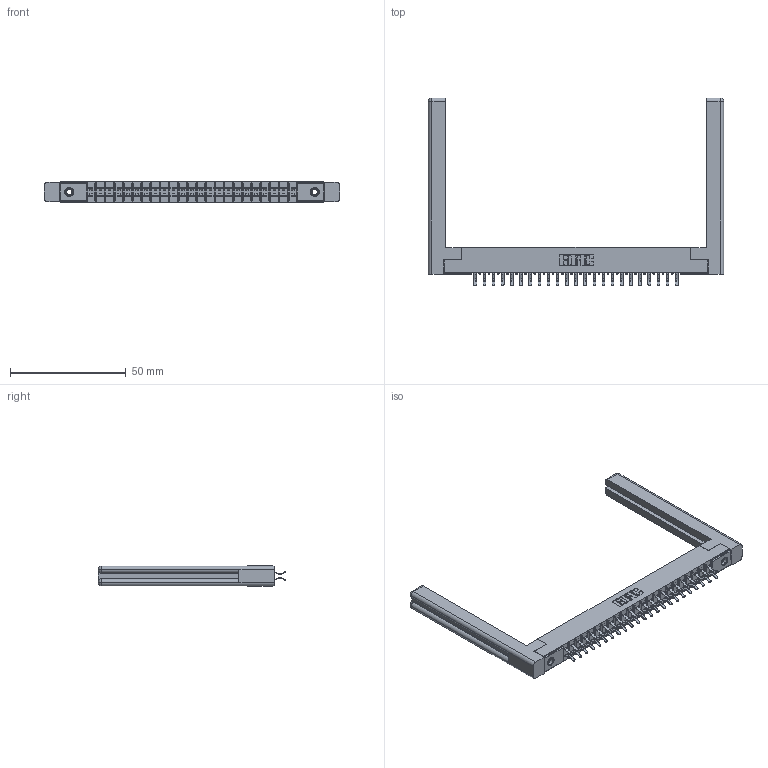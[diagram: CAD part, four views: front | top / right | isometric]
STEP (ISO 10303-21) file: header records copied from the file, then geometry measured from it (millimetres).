
FILE_DESCRIPTION (( 'STEP AP203' ), '1' );
FILE_NAME ('355-046-556-558.STEP', '2019-09-11T14:59:53', ( '' ), ( '' ), 'SwSTEP 2.0', 'SolidWorks 2016', '' );
FILE_SCHEMA (( 'CONFIG_CONTROL_DESIGN' ));
Length unit declared in the file: inch
Products named in the file (5): 345-250-001_345-250-001-102; 305 Part_.156 Dia; 355-046-556-558; 307-220-058; 305-290-001_556
Assembly tree (51 placements, depth 2):
  355-046-556-558
    305 Part_.156 Dia
    305-290-001_556  x46
    345-250-001_345-250-001-102  x2
    307-220-058  x2
Bounding box: 127.76 x 81.28 x 8.71 mm (x, y, z)
Volume: 15406.5 mm3; surface area: 20350.7 mm2
Topology: 51 solids, 51 shells, 2834 faces, 8099 edges, 5262 vertices
Faces by surface type: plane 1578, cylinder 1140, sphere 92, cone 12, torus 12
Entity records: 30071 total; most frequent: CARTESIAN_POINT 4994, ORIENTED_EDGE 4896, DIRECTION 4812, EDGE_CURVE 2448, LINE 1944, VECTOR 1944, VERTEX_POINT 1562, AXIS2_PLACEMENT_3D 1434
